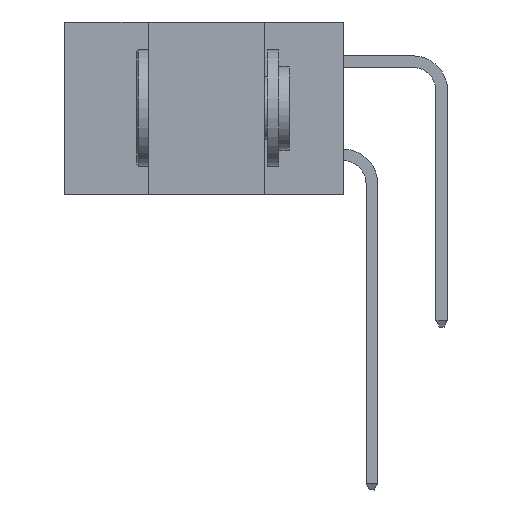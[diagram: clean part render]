
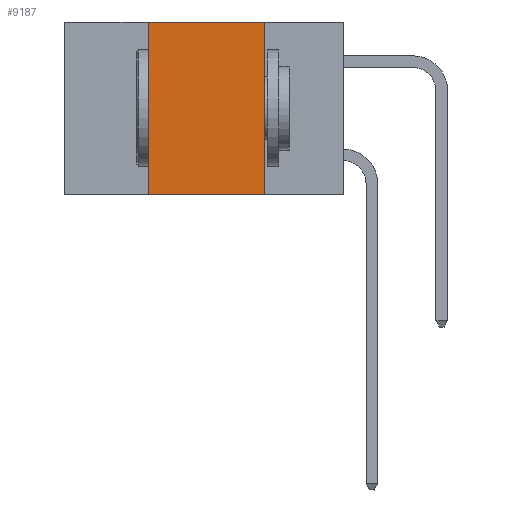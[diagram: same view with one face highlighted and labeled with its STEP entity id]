
A CAD part, left-side view. The second image highlights one B-rep face of the part: STEP entity #9187.
In plain terms, the highlighted planar face has unit normal (-1, 0, 0).
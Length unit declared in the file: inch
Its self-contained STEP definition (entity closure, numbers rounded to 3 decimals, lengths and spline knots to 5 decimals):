
#448 = EDGE_CURVE ( 'NONE', #4333, #3225, #12863, .T. ) ;
#499 = CARTESIAN_POINT ( 'NONE',  ( 0., 0.6, -0.37 ) ) ;
#1645 = VECTOR ( 'NONE', #6046, 39.37008 ) ;
#1896 = ORIENTED_EDGE ( 'NONE', *, *, #4240, .F. ) ;
#2049 = EDGE_LOOP ( 'NONE', ( #5837, #1896, #6542, #13626 ) ) ;
#2273 = DIRECTION ( 'NONE',  ( 0., 0., 1. ) ) ;
#2340 = DIRECTION ( 'NONE',  ( 0., -1., 0. ) ) ;
#3225 = VERTEX_POINT ( 'NONE', #4130 ) ;
#3313 = LINE ( 'NONE', #14618, #5576 ) ;
#3447 = LINE ( 'NONE', #4422, #14003 ) ;
#3598 = CARTESIAN_POINT ( 'NONE',  ( 0., 0.6, 0. ) ) ;
#4130 = CARTESIAN_POINT ( 'NONE',  ( 0., 0.17, -0.37 ) ) ;
#4240 = EDGE_CURVE ( 'NONE', #11223, #9748, #3447, .T. ) ;
#4333 = VERTEX_POINT ( 'NONE', #8292 ) ;
#4422 = CARTESIAN_POINT ( 'NONE',  ( 0., 0.6, 0. ) ) ;
#4730 = FACE_OUTER_BOUND ( 'NONE', #2049, .T. ) ;
#5576 = VECTOR ( 'NONE', #2273, 39.37008 ) ;
#5837 = ORIENTED_EDGE ( 'NONE', *, *, #10090, .F. ) ;
#6046 = DIRECTION ( 'NONE',  ( 0., -1., 0. ) ) ;
#6542 = ORIENTED_EDGE ( 'NONE', *, *, #9112, .F. ) ;
#7049 = CARTESIAN_POINT ( 'NONE',  ( 0., 0.42, 0. ) ) ;
#7113 = DIRECTION ( 'NONE',  ( 1., 0., 0. ) ) ;
#7262 = DIRECTION ( 'NONE',  ( 0., 0., -1. ) ) ;
#8292 = CARTESIAN_POINT ( 'NONE',  ( 0., 0.42, -0.37 ) ) ;
#8691 = CARTESIAN_POINT ( 'NONE',  ( 0., 0.17, 0. ) ) ;
#9112 = EDGE_CURVE ( 'NONE', #4333, #11223, #3313, .T. ) ;
#9187 = ADVANCED_FACE ( 'NONE', ( #4730 ), #13796, .F. ) ;
#9748 = VERTEX_POINT ( 'NONE', #8691 ) ;
#9835 = DIRECTION ( 'NONE',  ( 0., 0., -1. ) ) ;
#10090 = EDGE_CURVE ( 'NONE', #9748, #3225, #13180, .T. ) ;
#10281 = VECTOR ( 'NONE', #9835, 39.37008 ) ;
#11223 = VERTEX_POINT ( 'NONE', #7049 ) ;
#12132 = CARTESIAN_POINT ( 'NONE',  ( 0., 0.17, -0.37 ) ) ;
#12863 = LINE ( 'NONE', #499, #1645 ) ;
#13180 = LINE ( 'NONE', #12132, #10281 ) ;
#13626 = ORIENTED_EDGE ( 'NONE', *, *, #448, .T. ) ;
#13796 = PLANE ( 'NONE',  #13872 ) ;
#13872 = AXIS2_PLACEMENT_3D ( 'NONE', #3598, #7113, #7262 ) ;
#14003 = VECTOR ( 'NONE', #2340, 39.37008 ) ;
#14618 = CARTESIAN_POINT ( 'NONE',  ( 0., 0.42, -0.37 ) ) ;
